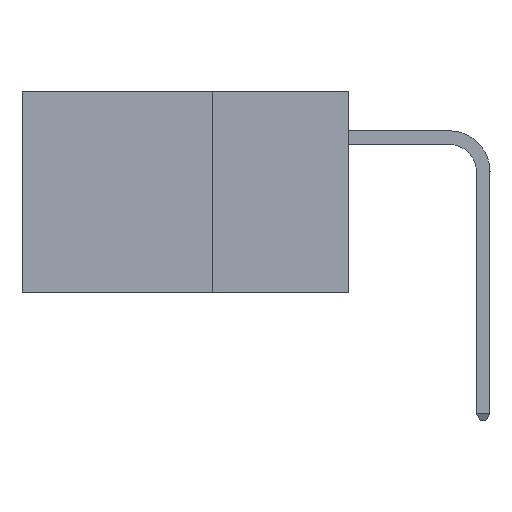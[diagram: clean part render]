
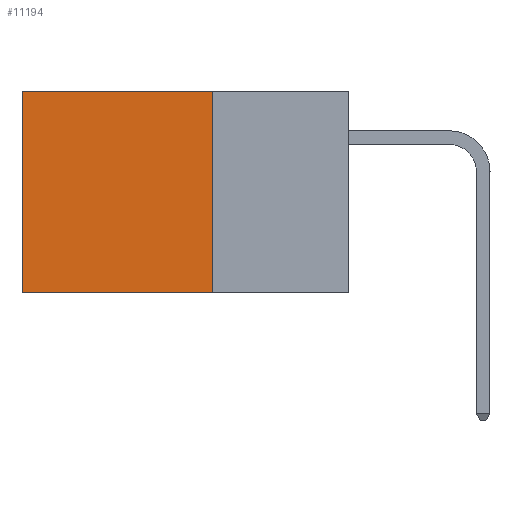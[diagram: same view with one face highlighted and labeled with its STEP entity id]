
A CAD part, left-side view. The second image highlights one B-rep face of the part: STEP entity #11194.
In plain terms, the highlighted planar face has unit normal (-1, 0, 0).
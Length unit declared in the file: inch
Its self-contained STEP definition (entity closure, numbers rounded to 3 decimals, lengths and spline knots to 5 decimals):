
#3917 = DIRECTION ( 'NONE',  ( 0., 1., 0. ) ) ;
#6001 = EDGE_LOOP ( 'NONE', ( #7140, #16275, #36583, #18948 ) ) ;
#6599 = EDGE_CURVE ( 'NONE', #37249, #33694, #40707, .T. ) ;
#7140 = ORIENTED_EDGE ( 'NONE', *, *, #25145, .T. ) ;
#7444 = CARTESIAN_POINT ( 'NONE',  ( 0.2875, 0.25, 0. ) ) ;
#8513 = DIRECTION ( 'NONE',  ( 0., 0., -1. ) ) ;
#11194 = ADVANCED_FACE ( 'NONE', ( #13388 ), #34612, .F. ) ;
#11279 = VERTEX_POINT ( 'NONE', #33226 ) ;
#11938 = CARTESIAN_POINT ( 'NONE',  ( 0.2875, 0.25, 0. ) ) ;
#12115 = DIRECTION ( 'NONE',  ( 0., 1., 0. ) ) ;
#13388 = FACE_OUTER_BOUND ( 'NONE', #6001, .T. ) ;
#13897 = VECTOR ( 'NONE', #12115, 39.37008 ) ;
#15946 = LINE ( 'NONE', #41899, #13897 ) ;
#16275 = ORIENTED_EDGE ( 'NONE', *, *, #38862, .F. ) ;
#17880 = CARTESIAN_POINT ( 'NONE',  ( 0.2875, 0.25, -0.37 ) ) ;
#17897 = LINE ( 'NONE', #39249, #27000 ) ;
#18618 = LINE ( 'NONE', #30866, #38990 ) ;
#18948 = ORIENTED_EDGE ( 'NONE', *, *, #32463, .T. ) ;
#21349 = VECTOR ( 'NONE', #22927, 39.37008 ) ;
#22927 = DIRECTION ( 'NONE',  ( 0., 0., -1. ) ) ;
#25145 = EDGE_CURVE ( 'NONE', #30783, #11279, #18618, .T. ) ;
#27000 = VECTOR ( 'NONE', #3917, 39.37008 ) ;
#28437 = DIRECTION ( 'NONE',  ( 1., 0., 0. ) ) ;
#29740 = CARTESIAN_POINT ( 'NONE',  ( 0.2875, 0.6, 0. ) ) ;
#30783 = VERTEX_POINT ( 'NONE', #29740 ) ;
#30866 = CARTESIAN_POINT ( 'NONE',  ( 0.2875, 0.6, 0. ) ) ;
#31720 = AXIS2_PLACEMENT_3D ( 'NONE', #11938, #28437, #41444 ) ;
#32463 = EDGE_CURVE ( 'NONE', #37249, #30783, #15946, .T. ) ;
#33226 = CARTESIAN_POINT ( 'NONE',  ( 0.2875, 0.6, -0.37 ) ) ;
#33694 = VERTEX_POINT ( 'NONE', #17880 ) ;
#34612 = PLANE ( 'NONE',  #31720 ) ;
#35350 = CARTESIAN_POINT ( 'NONE',  ( 0.2875, 0.25, 0. ) ) ;
#36583 = ORIENTED_EDGE ( 'NONE', *, *, #6599, .F. ) ;
#37249 = VERTEX_POINT ( 'NONE', #7444 ) ;
#38862 = EDGE_CURVE ( 'NONE', #33694, #11279, #17897, .T. ) ;
#38990 = VECTOR ( 'NONE', #8513, 39.37008 ) ;
#39249 = CARTESIAN_POINT ( 'NONE',  ( 0.2875, 0.25, -0.37 ) ) ;
#40707 = LINE ( 'NONE', #35350, #21349 ) ;
#41444 = DIRECTION ( 'NONE',  ( 0., 0., -1. ) ) ;
#41899 = CARTESIAN_POINT ( 'NONE',  ( 0.2875, 0.25, 0. ) ) ;
